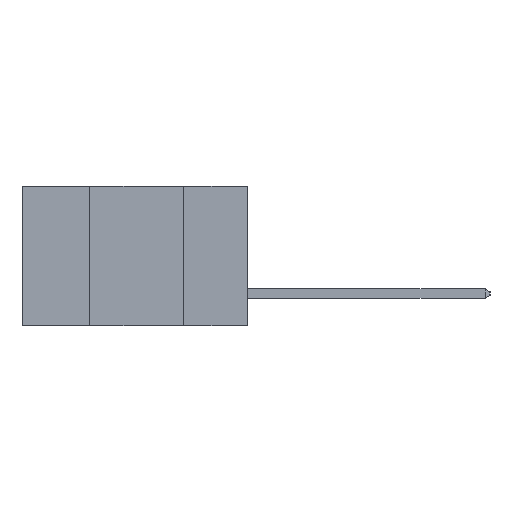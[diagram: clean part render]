
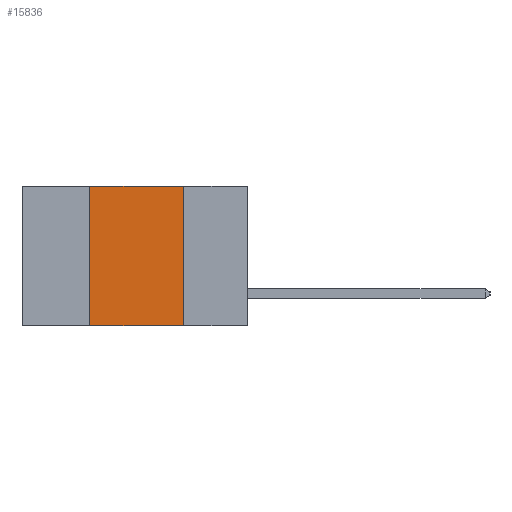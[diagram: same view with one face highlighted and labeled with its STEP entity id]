
A CAD part, left-side view. The second image highlights one B-rep face of the part: STEP entity #15836.
In plain terms, the highlighted planar face has unit normal (-1, 0, 0).
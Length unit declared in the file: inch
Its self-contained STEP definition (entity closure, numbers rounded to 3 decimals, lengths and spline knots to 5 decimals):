
#618 = VERTEX_POINT ( 'NONE', #2420 ) ;
#835 = VERTEX_POINT ( 'NONE', #15365 ) ;
#840 = EDGE_LOOP ( 'NONE', ( #6789, #14787, #4365, #9491 ) ) ;
#1091 = EDGE_CURVE ( 'NONE', #11381, #618, #6092, .T. ) ;
#1294 = LINE ( 'NONE', #4556, #16448 ) ;
#2038 = DIRECTION ( 'NONE',  ( 1., 0., 0. ) ) ;
#2252 = CARTESIAN_POINT ( 'NONE',  ( 0., 0.6, -0.37 ) ) ;
#2420 = CARTESIAN_POINT ( 'NONE',  ( 0., 0.17, -0.37 ) ) ;
#3076 = EDGE_CURVE ( 'NONE', #835, #17990, #14738, .T. ) ;
#3454 = PLANE ( 'NONE',  #7656 ) ;
#4236 = EDGE_CURVE ( 'NONE', #17990, #11381, #1294, .T. ) ;
#4365 = ORIENTED_EDGE ( 'NONE', *, *, #3076, .F. ) ;
#4556 = CARTESIAN_POINT ( 'NONE',  ( 0., 0.6, 0. ) ) ;
#4728 = CARTESIAN_POINT ( 'NONE',  ( 0., 0.17, 0. ) ) ;
#5163 = FACE_OUTER_BOUND ( 'NONE', #840, .T. ) ;
#6092 = LINE ( 'NONE', #4728, #12351 ) ;
#6789 = ORIENTED_EDGE ( 'NONE', *, *, #1091, .F. ) ;
#6867 = DIRECTION ( 'NONE',  ( 0., 0., -1. ) ) ;
#7656 = AXIS2_PLACEMENT_3D ( 'NONE', #10621, #2038, #12044 ) ;
#7736 = CARTESIAN_POINT ( 'NONE',  ( 0., 0.42, 0. ) ) ;
#9491 = ORIENTED_EDGE ( 'NONE', *, *, #12614, .T. ) ;
#10621 = CARTESIAN_POINT ( 'NONE',  ( 0., 0.6, 0. ) ) ;
#10760 = DIRECTION ( 'NONE',  ( 0., -1., 0. ) ) ;
#11015 = VECTOR ( 'NONE', #11972, 39.37008 ) ;
#11381 = VERTEX_POINT ( 'NONE', #13870 ) ;
#11599 = CARTESIAN_POINT ( 'NONE',  ( 0., 0.42, 0. ) ) ;
#11972 = DIRECTION ( 'NONE',  ( 0., 0., 1. ) ) ;
#12044 = DIRECTION ( 'NONE',  ( 0., 0., -1. ) ) ;
#12351 = VECTOR ( 'NONE', #6867, 39.37008 ) ;
#12614 = EDGE_CURVE ( 'NONE', #835, #618, #15653, .T. ) ;
#13870 = CARTESIAN_POINT ( 'NONE',  ( 0., 0.17, 0. ) ) ;
#14479 = DIRECTION ( 'NONE',  ( 0., -1., 0. ) ) ;
#14738 = LINE ( 'NONE', #11599, #11015 ) ;
#14759 = VECTOR ( 'NONE', #10760, 39.37008 ) ;
#14787 = ORIENTED_EDGE ( 'NONE', *, *, #4236, .F. ) ;
#15365 = CARTESIAN_POINT ( 'NONE',  ( 0., 0.42, -0.37 ) ) ;
#15653 = LINE ( 'NONE', #2252, #14759 ) ;
#15836 = ADVANCED_FACE ( 'NONE', ( #5163 ), #3454, .F. ) ;
#16448 = VECTOR ( 'NONE', #14479, 39.37008 ) ;
#17990 = VERTEX_POINT ( 'NONE', #7736 ) ;
